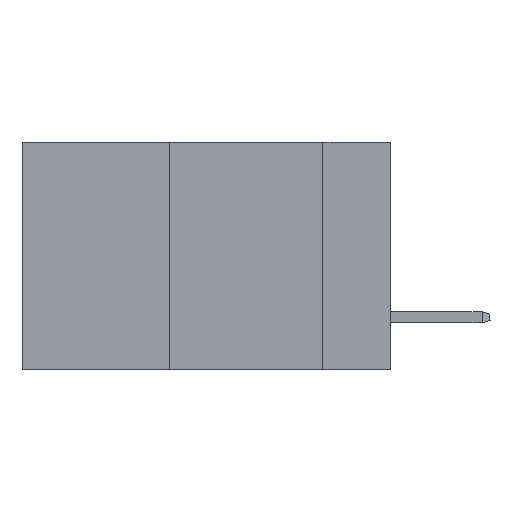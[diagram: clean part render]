
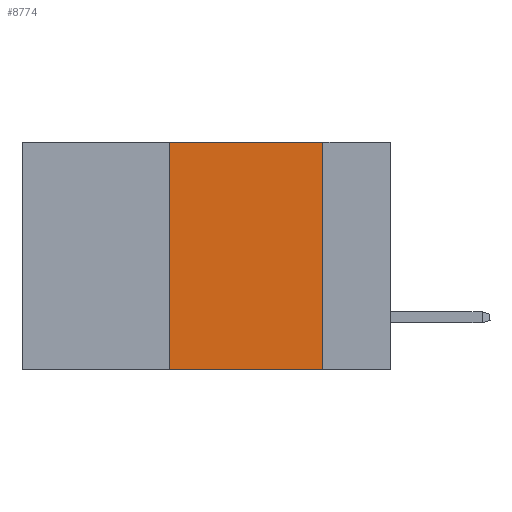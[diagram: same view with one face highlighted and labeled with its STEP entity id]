
A CAD part, left-side view. The second image highlights one B-rep face of the part: STEP entity #8774.
In plain terms, the highlighted planar face has unit normal (-1, 0, 0).
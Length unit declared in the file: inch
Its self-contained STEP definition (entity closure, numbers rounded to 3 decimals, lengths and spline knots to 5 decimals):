
#861 = DIRECTION ( 'NONE',  ( 0., 0., -1. ) ) ;
#1065 = AXIS2_PLACEMENT_3D ( 'NONE', #20294, #6888, #17354 ) ;
#1084 = VECTOR ( 'NONE', #39184, 39.37008 ) ;
#2035 = LINE ( 'NONE', #11988, #14179 ) ;
#5198 = DIRECTION ( 'NONE',  ( 0., 0., 1. ) ) ;
#5430 = LINE ( 'NONE', #21254, #28274 ) ;
#6888 = DIRECTION ( 'NONE',  ( 1., 0., 0. ) ) ;
#8774 = ADVANCED_FACE ( 'NONE', ( #33363 ), #40763, .F. ) ;
#9098 = LINE ( 'NONE', #34672, #1084 ) ;
#11089 = EDGE_CURVE ( 'NONE', #30572, #17885, #9098, .T. ) ;
#11788 = CARTESIAN_POINT ( 'NONE',  ( 0., 0.11, -0.37 ) ) ;
#11988 = CARTESIAN_POINT ( 'NONE',  ( 0., 0.36, 0. ) ) ;
#14179 = VECTOR ( 'NONE', #5198, 39.37008 ) ;
#17354 = DIRECTION ( 'NONE',  ( 0., 0., -1. ) ) ;
#17393 = CARTESIAN_POINT ( 'NONE',  ( 0., 0.11, 0. ) ) ;
#17885 = VERTEX_POINT ( 'NONE', #11788 ) ;
#17923 = ORIENTED_EDGE ( 'NONE', *, *, #22029, .F. ) ;
#19731 = DIRECTION ( 'NONE',  ( 0., -1., 0. ) ) ;
#19866 = ORIENTED_EDGE ( 'NONE', *, *, #32818, .F. ) ;
#20294 = CARTESIAN_POINT ( 'NONE',  ( 0., 0.6, 0. ) ) ;
#21254 = CARTESIAN_POINT ( 'NONE',  ( 0., 0.11, 0. ) ) ;
#22029 = EDGE_CURVE ( 'NONE', #40222, #44021, #30060, .T. ) ;
#22128 = ORIENTED_EDGE ( 'NONE', *, *, #11089, .T. ) ;
#24930 = CARTESIAN_POINT ( 'NONE',  ( 0., 0.36, -0.37 ) ) ;
#28274 = VECTOR ( 'NONE', #861, 39.37008 ) ;
#29453 = EDGE_LOOP ( 'NONE', ( #43465, #17923, #19866, #22128 ) ) ;
#29999 = CARTESIAN_POINT ( 'NONE',  ( 0., 0.6, 0. ) ) ;
#30060 = LINE ( 'NONE', #29999, #40780 ) ;
#30572 = VERTEX_POINT ( 'NONE', #24930 ) ;
#32818 = EDGE_CURVE ( 'NONE', #30572, #40222, #2035, .T. ) ;
#33363 = FACE_OUTER_BOUND ( 'NONE', #29453, .T. ) ;
#34672 = CARTESIAN_POINT ( 'NONE',  ( 0., 0.6, -0.37 ) ) ;
#39184 = DIRECTION ( 'NONE',  ( 0., -1., 0. ) ) ;
#40222 = VERTEX_POINT ( 'NONE', #42695 ) ;
#40763 = PLANE ( 'NONE',  #1065 ) ;
#40780 = VECTOR ( 'NONE', #19731, 39.37008 ) ;
#41687 = EDGE_CURVE ( 'NONE', #44021, #17885, #5430, .T. ) ;
#42695 = CARTESIAN_POINT ( 'NONE',  ( 0., 0.36, 0. ) ) ;
#43465 = ORIENTED_EDGE ( 'NONE', *, *, #41687, .F. ) ;
#44021 = VERTEX_POINT ( 'NONE', #17393 ) ;
